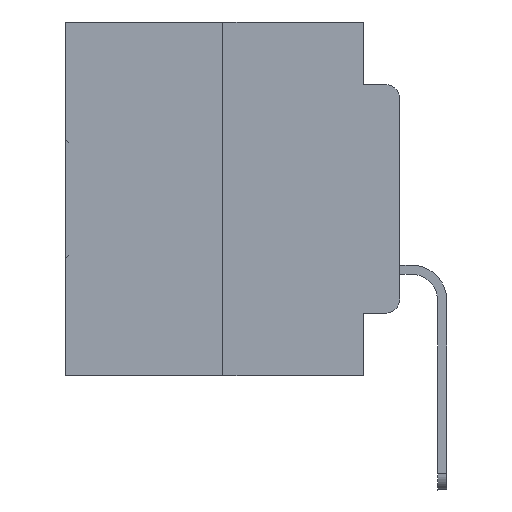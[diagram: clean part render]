
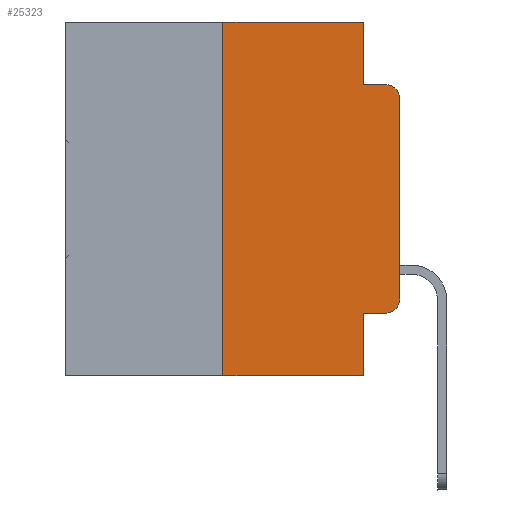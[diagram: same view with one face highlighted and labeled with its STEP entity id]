
A CAD part, left-side view. The second image highlights one B-rep face of the part: STEP entity #25323.
In plain terms, the highlighted planar face has unit normal (-1, 0, 0).
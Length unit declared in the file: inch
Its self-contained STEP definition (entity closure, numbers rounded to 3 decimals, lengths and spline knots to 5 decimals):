
#182 = EDGE_CURVE ( 'NONE', #10470, #23665, #27037, .T. ) ;
#378 = CARTESIAN_POINT ( 'NONE',  ( 0., 0.02, -0.4115 ) ) ;
#631 = EDGE_CURVE ( 'NONE', #6860, #10369, #25166, .T. ) ;
#692 = ORIENTED_EDGE ( 'NONE', *, *, #23854, .F. ) ;
#816 = VECTOR ( 'NONE', #9777, 39.37008 ) ;
#823 = EDGE_CURVE ( 'NONE', #12626, #12947, #23019, .T. ) ;
#960 = VERTEX_POINT ( 'NONE', #378 ) ;
#1424 = PLANE ( 'NONE',  #9194 ) ;
#2887 = VERTEX_POINT ( 'NONE', #20348 ) ;
#2911 = EDGE_CURVE ( 'NONE', #12947, #14913, #29538, .T. ) ;
#3081 = AXIS2_PLACEMENT_3D ( 'NONE', #14917, #21996, #29027 ) ;
#3187 = LINE ( 'NONE', #28872, #6342 ) ;
#3276 = DIRECTION ( 'NONE',  ( 1., 0., 0. ) ) ;
#3310 = ORIENTED_EDGE ( 'NONE', *, *, #19974, .T. ) ;
#3546 = VECTOR ( 'NONE', #6529, 39.37008 ) ;
#4439 = CARTESIAN_POINT ( 'NONE',  ( 0., 0.051, 0. ) ) ;
#4548 = VECTOR ( 'NONE', #8326, 39.37008 ) ;
#5007 = CARTESIAN_POINT ( 'NONE',  ( 0., 0.02, -0.0885 ) ) ;
#6079 = CARTESIAN_POINT ( 'NONE',  ( 0., 0.051, 0. ) ) ;
#6272 = DIRECTION ( 'NONE',  ( 0., -1., 0. ) ) ;
#6342 = VECTOR ( 'NONE', #12624, 39.37008 ) ;
#6529 = DIRECTION ( 'NONE',  ( 0., 0., -1. ) ) ;
#6709 = CARTESIAN_POINT ( 'NONE',  ( 0., 0.25, -0.5 ) ) ;
#6860 = VERTEX_POINT ( 'NONE', #6709 ) ;
#7748 = EDGE_CURVE ( 'NONE', #2887, #14913, #10352, .T. ) ;
#7877 = EDGE_CURVE ( 'NONE', #10470, #960, #24789, .T. ) ;
#7924 = VECTOR ( 'NONE', #6272, 39.37008 ) ;
#8045 = CARTESIAN_POINT ( 'NONE',  ( 0., 0.25, 0. ) ) ;
#8326 = DIRECTION ( 'NONE',  ( 0., 0., 1. ) ) ;
#8370 = EDGE_CURVE ( 'NONE', #960, #24850, #29441, .T. ) ;
#9194 = AXIS2_PLACEMENT_3D ( 'NONE', #17304, #3276, #26829 ) ;
#9777 = DIRECTION ( 'NONE',  ( 0., -1., 0. ) ) ;
#9803 = ORIENTED_EDGE ( 'NONE', *, *, #182, .F. ) ;
#10284 = VECTOR ( 'NONE', #10555, 39.37008 ) ;
#10352 = CIRCLE ( 'NONE', #19655, 0.02 ) ;
#10369 = VERTEX_POINT ( 'NONE', #8045 ) ;
#10470 = VERTEX_POINT ( 'NONE', #22699 ) ;
#10555 = DIRECTION ( 'NONE',  ( 0., -1., 0. ) ) ;
#10615 = CARTESIAN_POINT ( 'NONE',  ( 0., 0.25, 0. ) ) ;
#11673 = CARTESIAN_POINT ( 'NONE',  ( 0., 0.051, 0. ) ) ;
#12074 = DIRECTION ( 'NONE',  ( 0., 0., -1. ) ) ;
#12624 = DIRECTION ( 'NONE',  ( 0., -1., 0. ) ) ;
#12626 = VERTEX_POINT ( 'NONE', #4439 ) ;
#12947 = VERTEX_POINT ( 'NONE', #19581 ) ;
#13159 = LINE ( 'NONE', #15615, #29707 ) ;
#13917 = EDGE_LOOP ( 'NONE', ( #16024, #21142, #17522, #18010, #692, #21066, #3310, #9803, #19047, #22817 ) ) ;
#13974 = EDGE_CURVE ( 'NONE', #24850, #2887, #13159, .T. ) ;
#14913 = VERTEX_POINT ( 'NONE', #5007 ) ;
#14917 = CARTESIAN_POINT ( 'NONE',  ( 0., 0.02, -0.3915 ) ) ;
#15615 = CARTESIAN_POINT ( 'NONE',  ( 0., 0., 0. ) ) ;
#16024 = ORIENTED_EDGE ( 'NONE', *, *, #13974, .T. ) ;
#16343 = LINE ( 'NONE', #18966, #816 ) ;
#16967 = DIRECTION ( 'NONE',  ( -1., 0., 0. ) ) ;
#17304 = CARTESIAN_POINT ( 'NONE',  ( 0., 0.473, 0. ) ) ;
#17522 = ORIENTED_EDGE ( 'NONE', *, *, #2911, .F. ) ;
#17880 = CARTESIAN_POINT ( 'NONE',  ( 0., 0.051, -0.0885 ) ) ;
#18010 = ORIENTED_EDGE ( 'NONE', *, *, #823, .F. ) ;
#18966 = CARTESIAN_POINT ( 'NONE',  ( 0., 0.473, 0. ) ) ;
#19047 = ORIENTED_EDGE ( 'NONE', *, *, #7877, .T. ) ;
#19581 = CARTESIAN_POINT ( 'NONE',  ( 0., 0.051, -0.0885 ) ) ;
#19655 = AXIS2_PLACEMENT_3D ( 'NONE', #26488, #16967, #12074 ) ;
#19759 = CARTESIAN_POINT ( 'NONE',  ( 0., 0., -0.3915 ) ) ;
#19886 = CARTESIAN_POINT ( 'NONE',  ( 0., 0.051, -0.4115 ) ) ;
#19974 = EDGE_CURVE ( 'NONE', #6860, #23665, #3187, .T. ) ;
#20348 = CARTESIAN_POINT ( 'NONE',  ( 0., 0., -0.1085 ) ) ;
#20714 = DIRECTION ( 'NONE',  ( 0., 0., -1. ) ) ;
#21066 = ORIENTED_EDGE ( 'NONE', *, *, #631, .F. ) ;
#21142 = ORIENTED_EDGE ( 'NONE', *, *, #7748, .T. ) ;
#21996 = DIRECTION ( 'NONE',  ( -1., 0., 0. ) ) ;
#22699 = CARTESIAN_POINT ( 'NONE',  ( 0., 0.051, -0.4115 ) ) ;
#22817 = ORIENTED_EDGE ( 'NONE', *, *, #8370, .T. ) ;
#23019 = LINE ( 'NONE', #11673, #24480 ) ;
#23665 = VERTEX_POINT ( 'NONE', #25113 ) ;
#23854 = EDGE_CURVE ( 'NONE', #10369, #12626, #16343, .T. ) ;
#24480 = VECTOR ( 'NONE', #20714, 39.37008 ) ;
#24525 = FACE_OUTER_BOUND ( 'NONE', #13917, .T. ) ;
#24789 = LINE ( 'NONE', #19886, #7924 ) ;
#24850 = VERTEX_POINT ( 'NONE', #19759 ) ;
#25113 = CARTESIAN_POINT ( 'NONE',  ( 0., 0.051, -0.5 ) ) ;
#25166 = LINE ( 'NONE', #10615, #4548 ) ;
#25323 = ADVANCED_FACE ( 'NONE', ( #24525 ), #1424, .F. ) ;
#25441 = DIRECTION ( 'NONE',  ( 0., 0., 1. ) ) ;
#26488 = CARTESIAN_POINT ( 'NONE',  ( 0., 0.02, -0.1085 ) ) ;
#26829 = DIRECTION ( 'NONE',  ( 0., 0., -1. ) ) ;
#27037 = LINE ( 'NONE', #6079, #3546 ) ;
#28872 = CARTESIAN_POINT ( 'NONE',  ( 0., 0.473, -0.5 ) ) ;
#29027 = DIRECTION ( 'NONE',  ( 0., 0., -1. ) ) ;
#29441 = CIRCLE ( 'NONE', #3081, 0.02 ) ;
#29538 = LINE ( 'NONE', #17880, #10284 ) ;
#29707 = VECTOR ( 'NONE', #25441, 39.37008 ) ;
